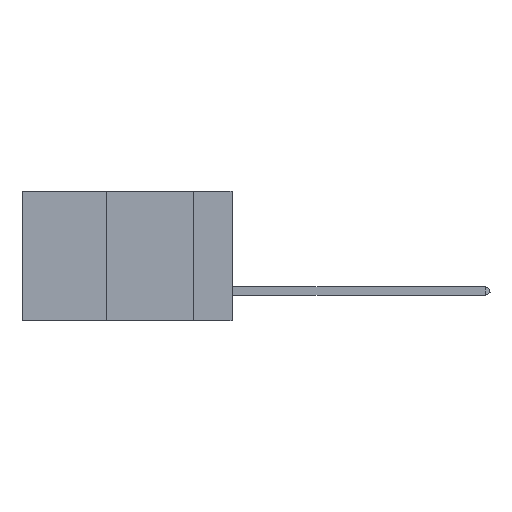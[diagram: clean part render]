
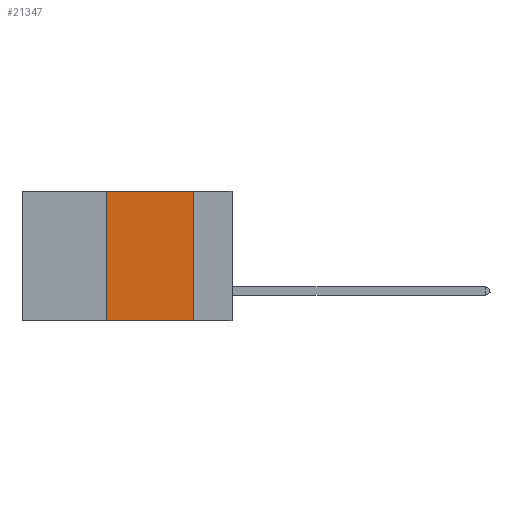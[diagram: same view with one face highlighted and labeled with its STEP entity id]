
A CAD part, left-side view. The second image highlights one B-rep face of the part: STEP entity #21347.
In plain terms, the highlighted planar face has unit normal (-1, 0, 0).
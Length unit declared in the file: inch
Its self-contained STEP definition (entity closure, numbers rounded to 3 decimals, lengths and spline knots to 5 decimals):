
#288 = CARTESIAN_POINT ( 'NONE',  ( 0., 0.6, 0. ) ) ;
#649 = DIRECTION ( 'NONE',  ( 1., 0., 0. ) ) ;
#1218 = ORIENTED_EDGE ( 'NONE', *, *, #6085, .T. ) ;
#1702 = CARTESIAN_POINT ( 'NONE',  ( 0., 0.36, 0. ) ) ;
#2707 = DIRECTION ( 'NONE',  ( 0., 0., -1. ) ) ;
#4290 = VECTOR ( 'NONE', #8111, 39.37008 ) ;
#4337 = LINE ( 'NONE', #4607, #17289 ) ;
#4607 = CARTESIAN_POINT ( 'NONE',  ( 0., 0.11, 0. ) ) ;
#4699 = AXIS2_PLACEMENT_3D ( 'NONE', #8752, #649, #24417 ) ;
#5245 = LINE ( 'NONE', #1702, #23805 ) ;
#5634 = VERTEX_POINT ( 'NONE', #16148 ) ;
#5767 = VECTOR ( 'NONE', #10475, 39.37008 ) ;
#5839 = VERTEX_POINT ( 'NONE', #12903 ) ;
#6085 = EDGE_CURVE ( 'NONE', #5839, #12617, #13747, .T. ) ;
#7016 = LINE ( 'NONE', #288, #4290 ) ;
#8111 = DIRECTION ( 'NONE',  ( 0., -1., 0. ) ) ;
#8752 = CARTESIAN_POINT ( 'NONE',  ( 0., 0.6, 0. ) ) ;
#10420 = ORIENTED_EDGE ( 'NONE', *, *, #19638, .F. ) ;
#10475 = DIRECTION ( 'NONE',  ( 0., -1., 0. ) ) ;
#12617 = VERTEX_POINT ( 'NONE', #19973 ) ;
#12903 = CARTESIAN_POINT ( 'NONE',  ( 0., 0.36, -0.37 ) ) ;
#13747 = LINE ( 'NONE', #20388, #5767 ) ;
#14871 = VERTEX_POINT ( 'NONE', #20426 ) ;
#15731 = DIRECTION ( 'NONE',  ( 0., 0., 1. ) ) ;
#16148 = CARTESIAN_POINT ( 'NONE',  ( 0., 0.11, 0. ) ) ;
#16604 = PLANE ( 'NONE',  #4699 ) ;
#17289 = VECTOR ( 'NONE', #2707, 39.37008 ) ;
#17857 = EDGE_CURVE ( 'NONE', #5839, #14871, #5245, .T. ) ;
#18046 = EDGE_CURVE ( 'NONE', #5634, #12617, #4337, .T. ) ;
#18592 = ORIENTED_EDGE ( 'NONE', *, *, #18046, .F. ) ;
#19582 = FACE_OUTER_BOUND ( 'NONE', #19880, .T. ) ;
#19638 = EDGE_CURVE ( 'NONE', #14871, #5634, #7016, .T. ) ;
#19880 = EDGE_LOOP ( 'NONE', ( #18592, #10420, #21658, #1218 ) ) ;
#19973 = CARTESIAN_POINT ( 'NONE',  ( 0., 0.11, -0.37 ) ) ;
#20388 = CARTESIAN_POINT ( 'NONE',  ( 0., 0.6, -0.37 ) ) ;
#20426 = CARTESIAN_POINT ( 'NONE',  ( 0., 0.36, 0. ) ) ;
#21347 = ADVANCED_FACE ( 'NONE', ( #19582 ), #16604, .F. ) ;
#21658 = ORIENTED_EDGE ( 'NONE', *, *, #17857, .F. ) ;
#23805 = VECTOR ( 'NONE', #15731, 39.37008 ) ;
#24417 = DIRECTION ( 'NONE',  ( 0., 0., -1. ) ) ;
